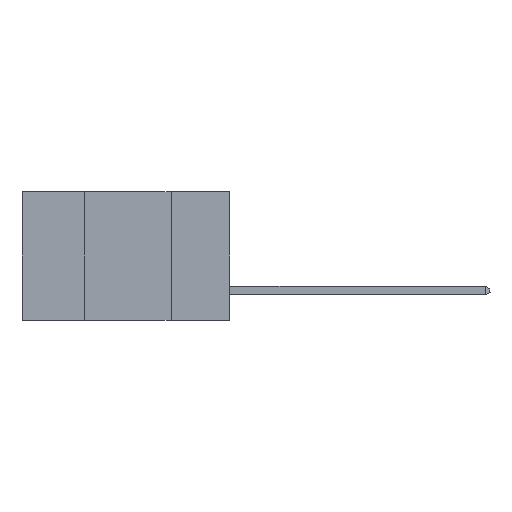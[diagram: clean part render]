
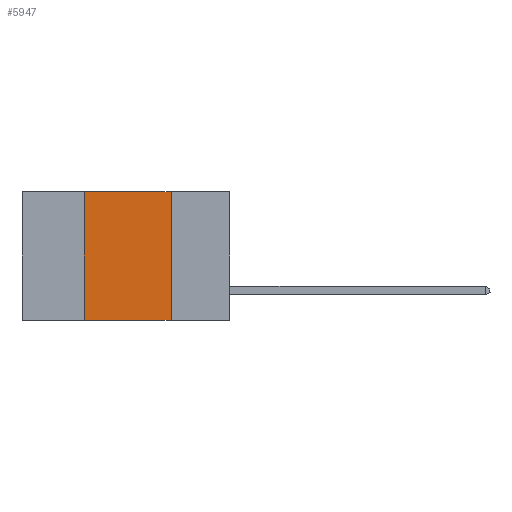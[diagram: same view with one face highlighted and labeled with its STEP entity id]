
A CAD part, left-side view. The second image highlights one B-rep face of the part: STEP entity #5947.
In plain terms, the highlighted planar face has unit normal (-1, 0, 0).
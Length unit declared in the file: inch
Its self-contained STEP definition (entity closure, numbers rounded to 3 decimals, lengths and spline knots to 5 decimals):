
#533 = DIRECTION ( 'NONE',  ( 0., 0., -1. ) ) ;
#851 = LINE ( 'NONE', #4533, #5431 ) ;
#1362 = ORIENTED_EDGE ( 'NONE', *, *, #9413, .F. ) ;
#1430 = CARTESIAN_POINT ( 'NONE',  ( 0., 0.17, 0. ) ) ;
#1482 = CARTESIAN_POINT ( 'NONE',  ( 0., 0.6, -0.37 ) ) ;
#1648 = CARTESIAN_POINT ( 'NONE',  ( 0., 0.6, 0. ) ) ;
#1877 = VERTEX_POINT ( 'NONE', #4821 ) ;
#1897 = VECTOR ( 'NONE', #6225, 39.37008 ) ;
#3472 = AXIS2_PLACEMENT_3D ( 'NONE', #1648, #6394, #7203 ) ;
#3634 = ORIENTED_EDGE ( 'NONE', *, *, #9582, .F. ) ;
#4000 = VERTEX_POINT ( 'NONE', #9570 ) ;
#4279 = LINE ( 'NONE', #5127, #7540 ) ;
#4457 = DIRECTION ( 'NONE',  ( 0., -1., 0. ) ) ;
#4485 = DIRECTION ( 'NONE',  ( 0., 0., 1. ) ) ;
#4489 = LINE ( 'NONE', #1482, #1897 ) ;
#4533 = CARTESIAN_POINT ( 'NONE',  ( 0., 0.6, 0. ) ) ;
#4821 = CARTESIAN_POINT ( 'NONE',  ( 0., 0.17, -0.37 ) ) ;
#4874 = EDGE_CURVE ( 'NONE', #6762, #1877, #4489, .T. ) ;
#5127 = CARTESIAN_POINT ( 'NONE',  ( 0., 0.17, 0. ) ) ;
#5159 = LINE ( 'NONE', #9183, #6921 ) ;
#5261 = ORIENTED_EDGE ( 'NONE', *, *, #9881, .F. ) ;
#5431 = VECTOR ( 'NONE', #4457, 39.37008 ) ;
#5947 = ADVANCED_FACE ( 'NONE', ( #9836 ), #7270, .F. ) ;
#6225 = DIRECTION ( 'NONE',  ( 0., -1., 0. ) ) ;
#6394 = DIRECTION ( 'NONE',  ( 1., 0., 0. ) ) ;
#6762 = VERTEX_POINT ( 'NONE', #8765 ) ;
#6921 = VECTOR ( 'NONE', #4485, 39.37008 ) ;
#7203 = DIRECTION ( 'NONE',  ( 0., 0., -1. ) ) ;
#7270 = PLANE ( 'NONE',  #3472 ) ;
#7271 = ORIENTED_EDGE ( 'NONE', *, *, #4874, .T. ) ;
#7540 = VECTOR ( 'NONE', #533, 39.37008 ) ;
#7898 = EDGE_LOOP ( 'NONE', ( #5261, #3634, #1362, #7271 ) ) ;
#8765 = CARTESIAN_POINT ( 'NONE',  ( 0., 0.42, -0.37 ) ) ;
#9183 = CARTESIAN_POINT ( 'NONE',  ( 0., 0.42, 0. ) ) ;
#9413 = EDGE_CURVE ( 'NONE', #6762, #4000, #5159, .T. ) ;
#9429 = VERTEX_POINT ( 'NONE', #1430 ) ;
#9570 = CARTESIAN_POINT ( 'NONE',  ( 0., 0.42, 0. ) ) ;
#9582 = EDGE_CURVE ( 'NONE', #4000, #9429, #851, .T. ) ;
#9836 = FACE_OUTER_BOUND ( 'NONE', #7898, .T. ) ;
#9881 = EDGE_CURVE ( 'NONE', #9429, #1877, #4279, .T. ) ;
